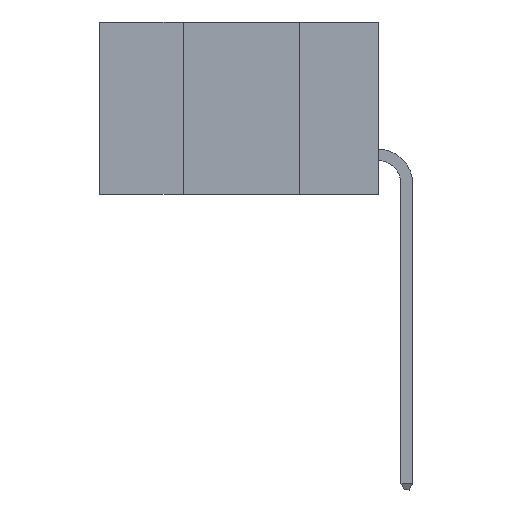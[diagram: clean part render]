
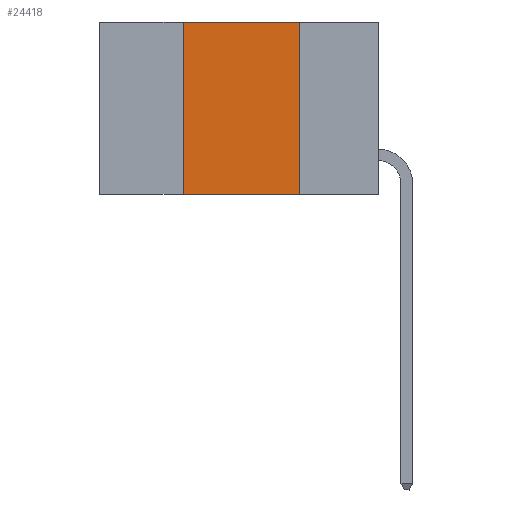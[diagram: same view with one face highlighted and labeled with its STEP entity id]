
A CAD part, left-side view. The second image highlights one B-rep face of the part: STEP entity #24418.
In plain terms, the highlighted planar face has unit normal (-1, 0, 0).
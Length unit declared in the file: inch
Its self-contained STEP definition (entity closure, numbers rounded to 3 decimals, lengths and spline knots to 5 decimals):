
#91 = FACE_OUTER_BOUND ( 'NONE', #17542, .T. ) ;
#1493 = DIRECTION ( 'NONE',  ( 0., 0., -1. ) ) ;
#3467 = DIRECTION ( 'NONE',  ( 0., 0., -1. ) ) ;
#4062 = VERTEX_POINT ( 'NONE', #8267 ) ;
#4476 = VERTEX_POINT ( 'NONE', #14372 ) ;
#5167 = CARTESIAN_POINT ( 'NONE',  ( 0., 0.6, 0. ) ) ;
#6041 = VERTEX_POINT ( 'NONE', #25069 ) ;
#6154 = DIRECTION ( 'NONE',  ( 0., -1., 0. ) ) ;
#7158 = DIRECTION ( 'NONE',  ( 0., -1., 0. ) ) ;
#8267 = CARTESIAN_POINT ( 'NONE',  ( 0., 0.42, 0. ) ) ;
#9344 = LINE ( 'NONE', #5167, #13957 ) ;
#10020 = LINE ( 'NONE', #17237, #15193 ) ;
#11532 = ORIENTED_EDGE ( 'NONE', *, *, #24431, .F. ) ;
#11796 = ORIENTED_EDGE ( 'NONE', *, *, #18693, .F. ) ;
#13015 = VECTOR ( 'NONE', #6154, 39.37008 ) ;
#13347 = CARTESIAN_POINT ( 'NONE',  ( 0., 0.6, 0. ) ) ;
#13637 = ORIENTED_EDGE ( 'NONE', *, *, #14177, .F. ) ;
#13957 = VECTOR ( 'NONE', #7158, 39.37008 ) ;
#14177 = EDGE_CURVE ( 'NONE', #4062, #4476, #9344, .T. ) ;
#14259 = LINE ( 'NONE', #23352, #23298 ) ;
#14372 = CARTESIAN_POINT ( 'NONE',  ( 0., 0.17, 0. ) ) ;
#14832 = EDGE_CURVE ( 'NONE', #6041, #19626, #22653, .T. ) ;
#14914 = AXIS2_PLACEMENT_3D ( 'NONE', #13347, #15272, #3467 ) ;
#15193 = VECTOR ( 'NONE', #1493, 39.37008 ) ;
#15272 = DIRECTION ( 'NONE',  ( 1., 0., 0. ) ) ;
#16582 = CARTESIAN_POINT ( 'NONE',  ( 0., 0.17, -0.37 ) ) ;
#17237 = CARTESIAN_POINT ( 'NONE',  ( 0., 0.17, 0. ) ) ;
#17542 = EDGE_LOOP ( 'NONE', ( #11532, #13637, #11796, #17765 ) ) ;
#17765 = ORIENTED_EDGE ( 'NONE', *, *, #14832, .T. ) ;
#17944 = CARTESIAN_POINT ( 'NONE',  ( 0., 0.6, -0.37 ) ) ;
#18693 = EDGE_CURVE ( 'NONE', #6041, #4062, #14259, .T. ) ;
#19626 = VERTEX_POINT ( 'NONE', #16582 ) ;
#22653 = LINE ( 'NONE', #17944, #13015 ) ;
#23298 = VECTOR ( 'NONE', #25273, 39.37008 ) ;
#23352 = CARTESIAN_POINT ( 'NONE',  ( 0., 0.42, 0. ) ) ;
#24418 = ADVANCED_FACE ( 'NONE', ( #91 ), #24896, .F. ) ;
#24431 = EDGE_CURVE ( 'NONE', #4476, #19626, #10020, .T. ) ;
#24896 = PLANE ( 'NONE',  #14914 ) ;
#25069 = CARTESIAN_POINT ( 'NONE',  ( 0., 0.42, -0.37 ) ) ;
#25273 = DIRECTION ( 'NONE',  ( 0., 0., 1. ) ) ;
